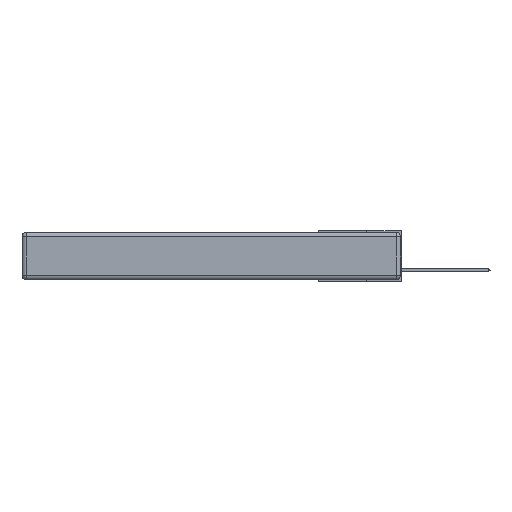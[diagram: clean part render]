
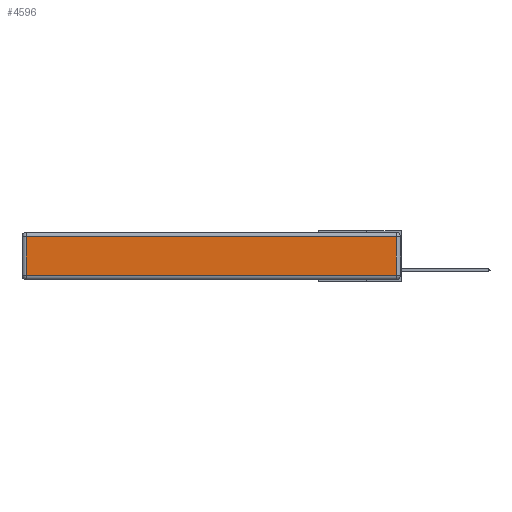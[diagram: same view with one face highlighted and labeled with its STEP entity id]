
A CAD part, left-side view. The second image highlights one B-rep face of the part: STEP entity #4596.
In plain terms, the highlighted planar face has unit normal (-1, 0, 0).
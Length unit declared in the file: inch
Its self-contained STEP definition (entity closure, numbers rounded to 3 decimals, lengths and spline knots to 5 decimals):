
#209 = PLANE ( 'NONE',  #7656 ) ;
#305 = EDGE_CURVE ( 'NONE', #20312, #12357, #22223, .T. ) ;
#4290 = CARTESIAN_POINT ( 'NONE',  ( 0., 0.03, -0.313 ) ) ;
#4324 = DIRECTION ( 'NONE',  ( 0., 1., 0. ) ) ;
#4433 = VECTOR ( 'NONE', #19020, 39.37008 ) ;
#4490 = DIRECTION ( 'NONE',  ( 0., 0., 1. ) ) ;
#4596 = ADVANCED_FACE ( 'NONE', ( #17168 ), #209, .T. ) ;
#6068 = CARTESIAN_POINT ( 'NONE',  ( 0., 2.72, -0.343 ) ) ;
#6197 = CARTESIAN_POINT ( 'NONE',  ( 0., 2.75, -0.03 ) ) ;
#6644 = CARTESIAN_POINT ( 'NONE',  ( 0., 0.03, -0.343 ) ) ;
#7656 = AXIS2_PLACEMENT_3D ( 'NONE', #8464, #8908, #23275 ) ;
#7760 = LINE ( 'NONE', #6644, #24158 ) ;
#8464 = CARTESIAN_POINT ( 'NONE',  ( 0., 0., -0.343 ) ) ;
#8908 = DIRECTION ( 'NONE',  ( -1., 0., 0. ) ) ;
#10122 = ORIENTED_EDGE ( 'NONE', *, *, #12892, .T. ) ;
#11122 = ORIENTED_EDGE ( 'NONE', *, *, #21806, .T. ) ;
#11279 = VECTOR ( 'NONE', #16180, 39.37008 ) ;
#11594 = LINE ( 'NONE', #6197, #13848 ) ;
#12357 = VERTEX_POINT ( 'NONE', #23717 ) ;
#12892 = EDGE_CURVE ( 'NONE', #12357, #22097, #26342, .T. ) ;
#13181 = CARTESIAN_POINT ( 'NONE',  ( 0., 0., -0.313 ) ) ;
#13848 = VECTOR ( 'NONE', #4324, 39.37008 ) ;
#14790 = ORIENTED_EDGE ( 'NONE', *, *, #22379, .T. ) ;
#16180 = DIRECTION ( 'NONE',  ( 0., 0., -1. ) ) ;
#17168 = FACE_OUTER_BOUND ( 'NONE', #18918, .T. ) ;
#18918 = EDGE_LOOP ( 'NONE', ( #10122, #11122, #14790, #18992 ) ) ;
#18992 = ORIENTED_EDGE ( 'NONE', *, *, #305, .T. ) ;
#19020 = DIRECTION ( 'NONE',  ( 0., -1., 0. ) ) ;
#20312 = VERTEX_POINT ( 'NONE', #24741 ) ;
#21806 = EDGE_CURVE ( 'NONE', #22097, #24676, #7760, .T. ) ;
#22097 = VERTEX_POINT ( 'NONE', #4290 ) ;
#22223 = LINE ( 'NONE', #6068, #11279 ) ;
#22379 = EDGE_CURVE ( 'NONE', #24676, #20312, #11594, .T. ) ;
#22427 = CARTESIAN_POINT ( 'NONE',  ( 0., 0.03, -0.03 ) ) ;
#23275 = DIRECTION ( 'NONE',  ( 0., 0., 1. ) ) ;
#23717 = CARTESIAN_POINT ( 'NONE',  ( 0., 2.72, -0.313 ) ) ;
#24158 = VECTOR ( 'NONE', #4490, 39.37008 ) ;
#24676 = VERTEX_POINT ( 'NONE', #22427 ) ;
#24741 = CARTESIAN_POINT ( 'NONE',  ( 0., 2.72, -0.03 ) ) ;
#26342 = LINE ( 'NONE', #13181, #4433 ) ;
